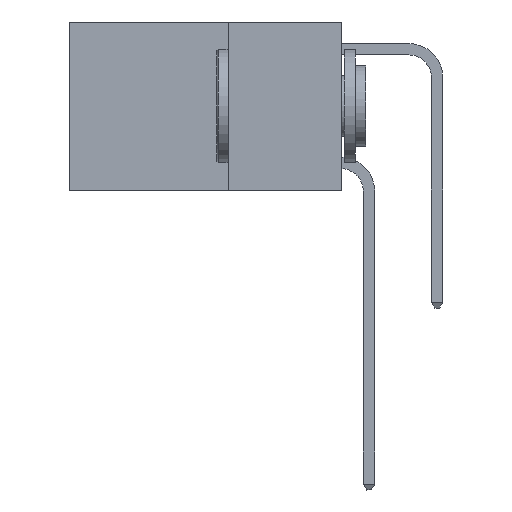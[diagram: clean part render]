
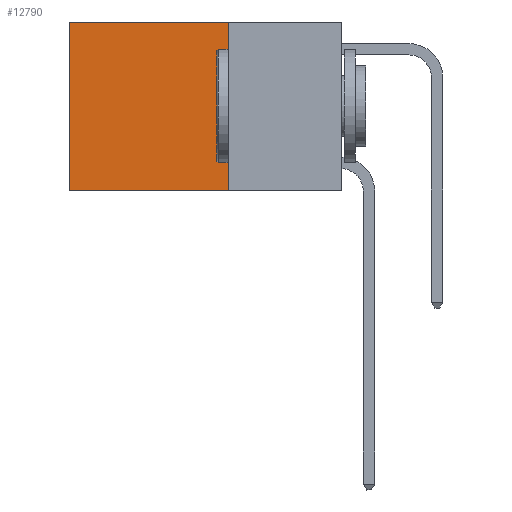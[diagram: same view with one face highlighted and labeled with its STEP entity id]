
A CAD part, left-side view. The second image highlights one B-rep face of the part: STEP entity #12790.
In plain terms, the highlighted planar face has unit normal (-1, 0, 0).
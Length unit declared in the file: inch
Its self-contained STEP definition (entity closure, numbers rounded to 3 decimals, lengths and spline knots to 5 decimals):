
#363 = VECTOR ( 'NONE', #2160, 39.37008 ) ;
#526 = VECTOR ( 'NONE', #20507, 39.37008 ) ;
#950 = EDGE_CURVE ( 'NONE', #15477, #18617, #7670, .T. ) ;
#1294 = EDGE_CURVE ( 'NONE', #21595, #18617, #7640, .T. ) ;
#2160 = DIRECTION ( 'NONE',  ( 0., 0., -1. ) ) ;
#2186 = DIRECTION ( 'NONE',  ( 0., 1., 0. ) ) ;
#2896 = EDGE_CURVE ( 'NONE', #10570, #21595, #18579, .T. ) ;
#3977 = LINE ( 'NONE', #10925, #10790 ) ;
#4475 = EDGE_CURVE ( 'NONE', #10570, #15477, #3977, .T. ) ;
#6923 = ORIENTED_EDGE ( 'NONE', *, *, #1294, .T. ) ;
#7640 = LINE ( 'NONE', #14471, #363 ) ;
#7670 = LINE ( 'NONE', #21681, #18406 ) ;
#7776 = CARTESIAN_POINT ( 'NONE',  ( 0.2625, 0.25, -0.37 ) ) ;
#7862 = DIRECTION ( 'NONE',  ( 0., 0., -1. ) ) ;
#10570 = VERTEX_POINT ( 'NONE', #17131 ) ;
#10719 = FACE_OUTER_BOUND ( 'NONE', #11582, .T. ) ;
#10790 = VECTOR ( 'NONE', #21186, 39.37008 ) ;
#10925 = CARTESIAN_POINT ( 'NONE',  ( 0.2625, 0.25, 0. ) ) ;
#11582 = EDGE_LOOP ( 'NONE', ( #6923, #17974, #13995, #20980 ) ) ;
#11629 = CARTESIAN_POINT ( 'NONE',  ( 0.2625, 0.6, 0. ) ) ;
#12790 = ADVANCED_FACE ( 'NONE', ( #10719 ), #17659, .F. ) ;
#13228 = DIRECTION ( 'NONE',  ( 1., 0., 0. ) ) ;
#13685 = CARTESIAN_POINT ( 'NONE',  ( 0.2625, 0.6, -0.37 ) ) ;
#13753 = AXIS2_PLACEMENT_3D ( 'NONE', #21869, #13228, #7862 ) ;
#13995 = ORIENTED_EDGE ( 'NONE', *, *, #4475, .F. ) ;
#14471 = CARTESIAN_POINT ( 'NONE',  ( 0.2625, 0.6, 0. ) ) ;
#15477 = VERTEX_POINT ( 'NONE', #7776 ) ;
#16884 = CARTESIAN_POINT ( 'NONE',  ( 0.2625, 0.25, 0. ) ) ;
#17131 = CARTESIAN_POINT ( 'NONE',  ( 0.2625, 0.25, 0. ) ) ;
#17659 = PLANE ( 'NONE',  #13753 ) ;
#17974 = ORIENTED_EDGE ( 'NONE', *, *, #950, .F. ) ;
#18406 = VECTOR ( 'NONE', #2186, 39.37008 ) ;
#18579 = LINE ( 'NONE', #16884, #526 ) ;
#18617 = VERTEX_POINT ( 'NONE', #13685 ) ;
#20507 = DIRECTION ( 'NONE',  ( 0., 1., 0. ) ) ;
#20980 = ORIENTED_EDGE ( 'NONE', *, *, #2896, .T. ) ;
#21186 = DIRECTION ( 'NONE',  ( 0., 0., -1. ) ) ;
#21595 = VERTEX_POINT ( 'NONE', #11629 ) ;
#21681 = CARTESIAN_POINT ( 'NONE',  ( 0.2625, 0.25, -0.37 ) ) ;
#21869 = CARTESIAN_POINT ( 'NONE',  ( 0.2625, 0.25, 0. ) ) ;
